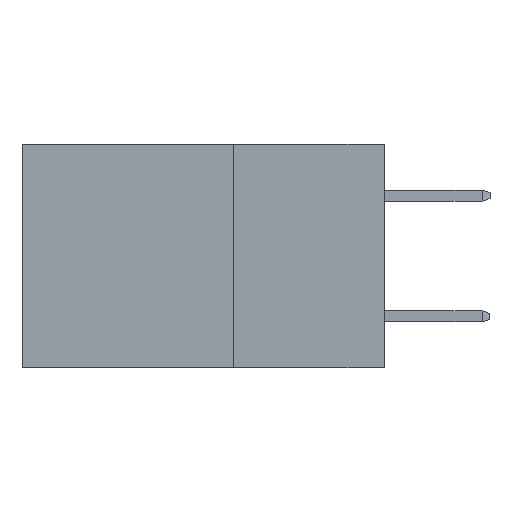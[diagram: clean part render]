
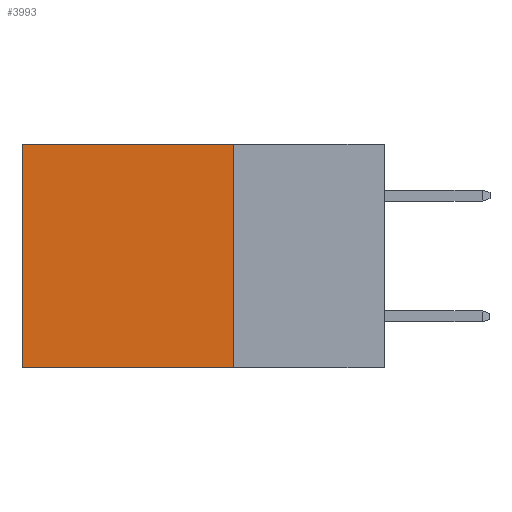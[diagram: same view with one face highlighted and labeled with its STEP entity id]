
A CAD part, left-side view. The second image highlights one B-rep face of the part: STEP entity #3993.
In plain terms, the highlighted planar face has unit normal (-1, 0, 0).
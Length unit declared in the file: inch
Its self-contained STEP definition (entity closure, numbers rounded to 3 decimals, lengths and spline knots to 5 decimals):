
#1243 = EDGE_CURVE ( 'NONE', #4424, #1885, #3790, .T. ) ;
#1624 = LINE ( 'NONE', #8870, #8436 ) ;
#1885 = VERTEX_POINT ( 'NONE', #11248 ) ;
#2089 = DIRECTION ( 'NONE',  ( 0., 0., -1. ) ) ;
#2126 = DIRECTION ( 'NONE',  ( 0., 0., -1. ) ) ;
#3294 = ORIENTED_EDGE ( 'NONE', *, *, #4422, .T. ) ;
#3319 = ORIENTED_EDGE ( 'NONE', *, *, #4699, .F. ) ;
#3366 = CARTESIAN_POINT ( 'NONE',  ( 0.298, 0.6, -0.37 ) ) ;
#3372 = ORIENTED_EDGE ( 'NONE', *, *, #1243, .F. ) ;
#3406 = ORIENTED_EDGE ( 'NONE', *, *, #8312, .T. ) ;
#3709 = CARTESIAN_POINT ( 'NONE',  ( 0.298, 0.25, 0. ) ) ;
#3790 = LINE ( 'NONE', #10708, #7953 ) ;
#3993 = ADVANCED_FACE ( 'NONE', ( #4097 ), #10866, .F. ) ;
#4097 = FACE_OUTER_BOUND ( 'NONE', #7431, .T. ) ;
#4422 = EDGE_CURVE ( 'NONE', #6730, #8509, #6356, .T. ) ;
#4424 = VERTEX_POINT ( 'NONE', #10125 ) ;
#4494 = DIRECTION ( 'NONE',  ( 1., 0., 0. ) ) ;
#4699 = EDGE_CURVE ( 'NONE', #1885, #8509, #9667, .T. ) ;
#5694 = CARTESIAN_POINT ( 'NONE',  ( 0.298, 0.25, -0.37 ) ) ;
#5983 = DIRECTION ( 'NONE',  ( 0., 1., 0. ) ) ;
#6017 = AXIS2_PLACEMENT_3D ( 'NONE', #3709, #4494, #2126 ) ;
#6356 = LINE ( 'NONE', #11243, #10293 ) ;
#6730 = VERTEX_POINT ( 'NONE', #8174 ) ;
#7431 = EDGE_LOOP ( 'NONE', ( #3294, #3319, #3372, #3406 ) ) ;
#7542 = VECTOR ( 'NONE', #5983, 39.37008 ) ;
#7953 = VECTOR ( 'NONE', #8758, 39.37008 ) ;
#8174 = CARTESIAN_POINT ( 'NONE',  ( 0.298, 0.6, 0. ) ) ;
#8312 = EDGE_CURVE ( 'NONE', #4424, #6730, #1624, .T. ) ;
#8436 = VECTOR ( 'NONE', #8559, 39.37008 ) ;
#8509 = VERTEX_POINT ( 'NONE', #3366 ) ;
#8559 = DIRECTION ( 'NONE',  ( 0., 1., 0. ) ) ;
#8758 = DIRECTION ( 'NONE',  ( 0., 0., -1. ) ) ;
#8870 = CARTESIAN_POINT ( 'NONE',  ( 0.298, 0.25, 0. ) ) ;
#9667 = LINE ( 'NONE', #5694, #7542 ) ;
#10125 = CARTESIAN_POINT ( 'NONE',  ( 0.298, 0.25, 0. ) ) ;
#10293 = VECTOR ( 'NONE', #2089, 39.37008 ) ;
#10708 = CARTESIAN_POINT ( 'NONE',  ( 0.298, 0.25, 0. ) ) ;
#10866 = PLANE ( 'NONE',  #6017 ) ;
#11243 = CARTESIAN_POINT ( 'NONE',  ( 0.298, 0.6, 0. ) ) ;
#11248 = CARTESIAN_POINT ( 'NONE',  ( 0.298, 0.25, -0.37 ) ) ;
